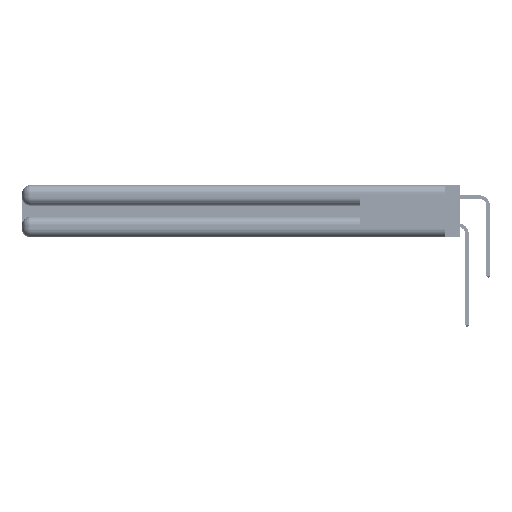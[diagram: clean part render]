
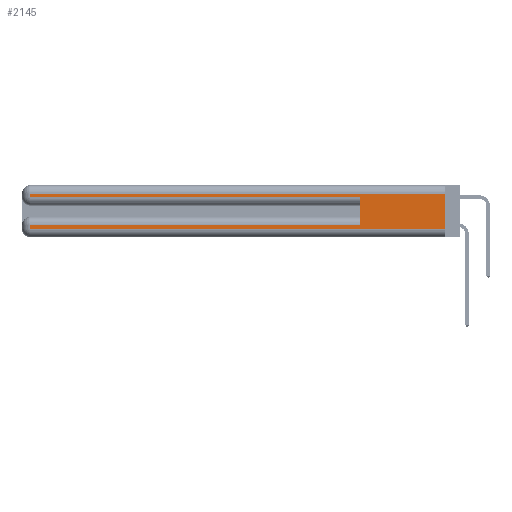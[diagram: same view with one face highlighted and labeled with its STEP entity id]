
A CAD part, left-side view. The second image highlights one B-rep face of the part: STEP entity #2145.
In plain terms, the highlighted planar face has unit normal (-1, 0, 0).
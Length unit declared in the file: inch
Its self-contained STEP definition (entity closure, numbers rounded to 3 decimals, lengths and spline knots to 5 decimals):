
#1041 = EDGE_CURVE ( 'NONE', #40869, #20267, #45171, .T. ) ;
#2145 = ADVANCED_FACE ( 'NONE', ( #45699 ), #31187, .F. ) ;
#4068 = CARTESIAN_POINT ( 'NONE',  ( 0., 0., 0.37 ) ) ;
#5387 = CARTESIAN_POINT ( 'NONE',  ( 0., 0., 0.37 ) ) ;
#5867 = CARTESIAN_POINT ( 'NONE',  ( 0., 2.94, 0.37 ) ) ;
#6930 = LINE ( 'NONE', #4068, #15777 ) ;
#7359 = DIRECTION ( 'NONE',  ( 0., 0., -1. ) ) ;
#8499 = AXIS2_PLACEMENT_3D ( 'NONE', #5387, #9754, #39717 ) ;
#9032 = CARTESIAN_POINT ( 'NONE',  ( 0., 2.94, 0.085 ) ) ;
#9640 = VECTOR ( 'NONE', #54543, 39.37008 ) ;
#9754 = DIRECTION ( 'NONE',  ( 1., 0., 0. ) ) ;
#9956 = DIRECTION ( 'NONE',  ( 0., 0., 1. ) ) ;
#10435 = DIRECTION ( 'NONE',  ( 0., 0., -1. ) ) ;
#11382 = VECTOR ( 'NONE', #9956, 39.37008 ) ;
#14650 = ORIENTED_EDGE ( 'NONE', *, *, #40566, .T. ) ;
#15132 = LINE ( 'NONE', #17342, #35174 ) ;
#15230 = EDGE_CURVE ( 'NONE', #52102, #43179, #41010, .T. ) ;
#15777 = VECTOR ( 'NONE', #38407, 39.37008 ) ;
#15842 = CARTESIAN_POINT ( 'NONE',  ( 0., 2.94, 0.31 ) ) ;
#17342 = CARTESIAN_POINT ( 'NONE',  ( 0., 0., 0.085 ) ) ;
#17993 = ORIENTED_EDGE ( 'NONE', *, *, #28847, .T. ) ;
#18108 = VECTOR ( 'NONE', #34320, 39.37008 ) ;
#20267 = VERTEX_POINT ( 'NONE', #40983 ) ;
#21710 = EDGE_CURVE ( 'NONE', #29626, #46069, #24130, .T. ) ;
#22016 = ORIENTED_EDGE ( 'NONE', *, *, #15230, .T. ) ;
#22636 = ORIENTED_EDGE ( 'NONE', *, *, #1041, .T. ) ;
#23861 = CARTESIAN_POINT ( 'NONE',  ( 0., 2.94, 0.06 ) ) ;
#24130 = LINE ( 'NONE', #31375, #11382 ) ;
#25728 = DIRECTION ( 'NONE',  ( 0., 1., 0. ) ) ;
#25792 = EDGE_LOOP ( 'NONE', ( #49964, #43980, #22636, #38007, #28023, #17993, #22016, #14650 ) ) ;
#27206 = CARTESIAN_POINT ( 'NONE',  ( 0., 0., 0.31 ) ) ;
#28023 = ORIENTED_EDGE ( 'NONE', *, *, #21710, .F. ) ;
#28847 = EDGE_CURVE ( 'NONE', #29626, #52102, #15132, .T. ) ;
#29381 = CARTESIAN_POINT ( 'NONE',  ( 0., 0., 0.06 ) ) ;
#29626 = VERTEX_POINT ( 'NONE', #33623 ) ;
#30075 = CARTESIAN_POINT ( 'NONE',  ( 0., 0., 0.31 ) ) ;
#30837 = LINE ( 'NONE', #30075, #18108 ) ;
#30876 = CARTESIAN_POINT ( 'NONE',  ( 0., 0., 0.06 ) ) ;
#31187 = PLANE ( 'NONE',  #8499 ) ;
#31375 = CARTESIAN_POINT ( 'NONE',  ( 0., 0.6, 0.145 ) ) ;
#32507 = VECTOR ( 'NONE', #10435, 39.37008 ) ;
#33623 = CARTESIAN_POINT ( 'NONE',  ( 0., 0.6, 0.085 ) ) ;
#33793 = LINE ( 'NONE', #50281, #9640 ) ;
#34211 = EDGE_CURVE ( 'NONE', #20267, #46069, #33793, .T. ) ;
#34320 = DIRECTION ( 'NONE',  ( 0., 1., 0. ) ) ;
#34493 = CARTESIAN_POINT ( 'NONE',  ( 0., 0.6, 0.285 ) ) ;
#35115 = DIRECTION ( 'NONE',  ( 0., -1., 0. ) ) ;
#35174 = VECTOR ( 'NONE', #25728, 39.37008 ) ;
#35393 = LINE ( 'NONE', #30876, #46701 ) ;
#36720 = VERTEX_POINT ( 'NONE', #29381 ) ;
#37192 = CARTESIAN_POINT ( 'NONE',  ( 0., 2.94, 0.37 ) ) ;
#38007 = ORIENTED_EDGE ( 'NONE', *, *, #34211, .T. ) ;
#38407 = DIRECTION ( 'NONE',  ( 0., 0., -1. ) ) ;
#39668 = VECTOR ( 'NONE', #7359, 39.37008 ) ;
#39717 = DIRECTION ( 'NONE',  ( 0., 0., -1. ) ) ;
#40566 = EDGE_CURVE ( 'NONE', #43179, #36720, #35393, .T. ) ;
#40869 = VERTEX_POINT ( 'NONE', #15842 ) ;
#40983 = CARTESIAN_POINT ( 'NONE',  ( 0., 2.94, 0.285 ) ) ;
#41010 = LINE ( 'NONE', #37192, #39668 ) ;
#43179 = VERTEX_POINT ( 'NONE', #23861 ) ;
#43503 = EDGE_CURVE ( 'NONE', #46248, #40869, #30837, .T. ) ;
#43980 = ORIENTED_EDGE ( 'NONE', *, *, #43503, .T. ) ;
#45171 = LINE ( 'NONE', #5867, #32507 ) ;
#45699 = FACE_OUTER_BOUND ( 'NONE', #25792, .T. ) ;
#46012 = EDGE_CURVE ( 'NONE', #46248, #36720, #6930, .T. ) ;
#46069 = VERTEX_POINT ( 'NONE', #34493 ) ;
#46248 = VERTEX_POINT ( 'NONE', #27206 ) ;
#46701 = VECTOR ( 'NONE', #35115, 39.37008 ) ;
#49964 = ORIENTED_EDGE ( 'NONE', *, *, #46012, .F. ) ;
#50281 = CARTESIAN_POINT ( 'NONE',  ( 0., 0., 0.285 ) ) ;
#52102 = VERTEX_POINT ( 'NONE', #9032 ) ;
#54543 = DIRECTION ( 'NONE',  ( 0., -1., 0. ) ) ;
